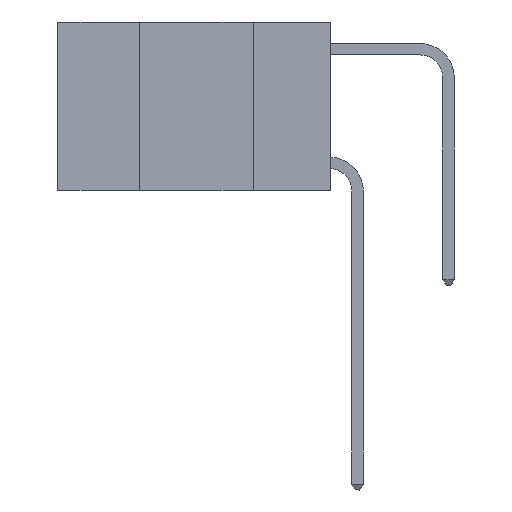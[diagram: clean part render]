
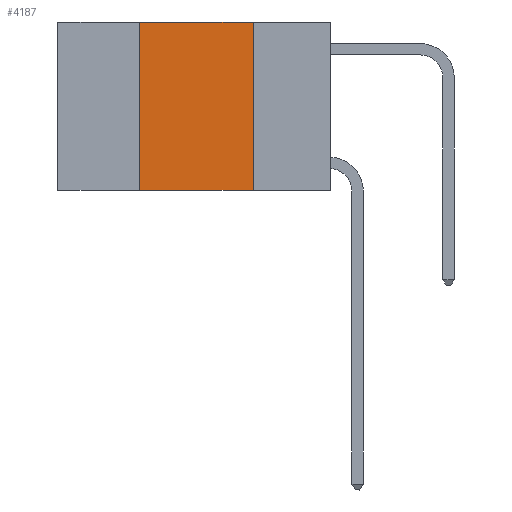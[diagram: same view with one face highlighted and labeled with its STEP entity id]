
A CAD part, left-side view. The second image highlights one B-rep face of the part: STEP entity #4187.
In plain terms, the highlighted planar face has unit normal (-1, 0, 0).
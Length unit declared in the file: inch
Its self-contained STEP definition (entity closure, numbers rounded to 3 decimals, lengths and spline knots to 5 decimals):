
#903 = EDGE_LOOP ( 'NONE', ( #3229, #9443, #6033, #5137 ) ) ;
#1241 = CARTESIAN_POINT ( 'NONE',  ( 0., 0.42, 0. ) ) ;
#1688 = DIRECTION ( 'NONE',  ( 0., -1., 0. ) ) ;
#2446 = EDGE_CURVE ( 'NONE', #14481, #10267, #9840, .T. ) ;
#2507 = AXIS2_PLACEMENT_3D ( 'NONE', #14035, #14381, #7434 ) ;
#2831 = VECTOR ( 'NONE', #11867, 39.37008 ) ;
#2933 = LINE ( 'NONE', #14735, #5889 ) ;
#3229 = ORIENTED_EDGE ( 'NONE', *, *, #4509, .F. ) ;
#4010 = DIRECTION ( 'NONE',  ( 0., -1., 0. ) ) ;
#4187 = ADVANCED_FACE ( 'NONE', ( #5383 ), #4558, .F. ) ;
#4216 = CARTESIAN_POINT ( 'NONE',  ( 0., 0.42, 0. ) ) ;
#4509 = EDGE_CURVE ( 'NONE', #4922, #5863, #9130, .T. ) ;
#4558 = PLANE ( 'NONE',  #2507 ) ;
#4922 = VERTEX_POINT ( 'NONE', #9827 ) ;
#5137 = ORIENTED_EDGE ( 'NONE', *, *, #16374, .T. ) ;
#5383 = FACE_OUTER_BOUND ( 'NONE', #903, .T. ) ;
#5440 = CARTESIAN_POINT ( 'NONE',  ( 0., 0.42, -0.37 ) ) ;
#5863 = VERTEX_POINT ( 'NONE', #9952 ) ;
#5889 = VECTOR ( 'NONE', #4010, 39.37008 ) ;
#6033 = ORIENTED_EDGE ( 'NONE', *, *, #2446, .F. ) ;
#7434 = DIRECTION ( 'NONE',  ( 0., 0., -1. ) ) ;
#8588 = CARTESIAN_POINT ( 'NONE',  ( 0., 0.6, -0.37 ) ) ;
#9130 = LINE ( 'NONE', #13046, #2831 ) ;
#9143 = VECTOR ( 'NONE', #1688, 39.37008 ) ;
#9443 = ORIENTED_EDGE ( 'NONE', *, *, #13285, .F. ) ;
#9827 = CARTESIAN_POINT ( 'NONE',  ( 0., 0.17, 0. ) ) ;
#9840 = LINE ( 'NONE', #1241, #15337 ) ;
#9952 = CARTESIAN_POINT ( 'NONE',  ( 0., 0.17, -0.37 ) ) ;
#10267 = VERTEX_POINT ( 'NONE', #4216 ) ;
#11867 = DIRECTION ( 'NONE',  ( 0., 0., -1. ) ) ;
#11981 = DIRECTION ( 'NONE',  ( 0., 0., 1. ) ) ;
#13046 = CARTESIAN_POINT ( 'NONE',  ( 0., 0.17, 0. ) ) ;
#13155 = LINE ( 'NONE', #8588, #9143 ) ;
#13285 = EDGE_CURVE ( 'NONE', #10267, #4922, #2933, .T. ) ;
#14035 = CARTESIAN_POINT ( 'NONE',  ( 0., 0.6, 0. ) ) ;
#14381 = DIRECTION ( 'NONE',  ( 1., 0., 0. ) ) ;
#14481 = VERTEX_POINT ( 'NONE', #5440 ) ;
#14735 = CARTESIAN_POINT ( 'NONE',  ( 0., 0.6, 0. ) ) ;
#15337 = VECTOR ( 'NONE', #11981, 39.37008 ) ;
#16374 = EDGE_CURVE ( 'NONE', #14481, #5863, #13155, .T. ) ;
